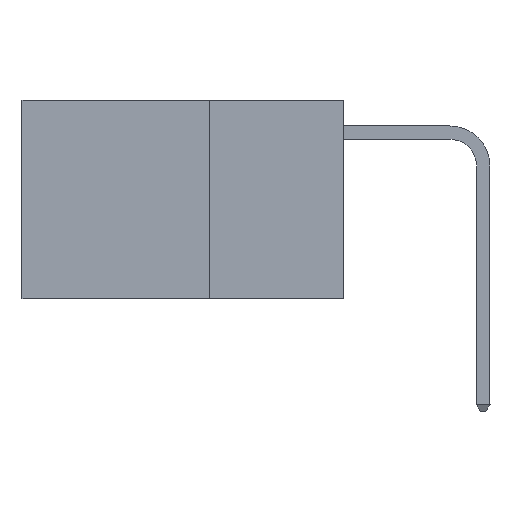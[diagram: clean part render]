
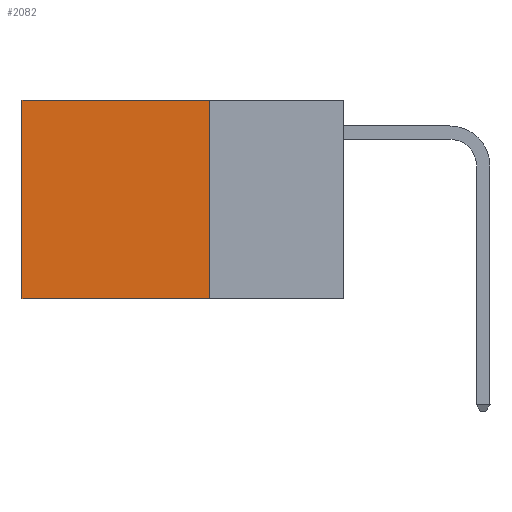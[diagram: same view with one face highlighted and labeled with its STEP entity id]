
A CAD part, left-side view. The second image highlights one B-rep face of the part: STEP entity #2082.
In plain terms, the highlighted planar face has unit normal (-1, 0, 0).
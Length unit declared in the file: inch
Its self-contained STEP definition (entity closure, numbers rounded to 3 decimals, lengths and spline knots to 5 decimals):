
#79 = EDGE_LOOP ( 'NONE', ( #1458, #371, #5404, #11312 ) ) ;
#185 = VECTOR ( 'NONE', #7376, 39.37008 ) ;
#190 = DIRECTION ( 'NONE',  ( 0., 1., 0. ) ) ;
#327 = LINE ( 'NONE', #8864, #5512 ) ;
#371 = ORIENTED_EDGE ( 'NONE', *, *, #4762, .F. ) ;
#1458 = ORIENTED_EDGE ( 'NONE', *, *, #11889, .T. ) ;
#1567 = CARTESIAN_POINT ( 'NONE',  ( 0.2625, 0.6, -0.37 ) ) ;
#1612 = EDGE_CURVE ( 'NONE', #6761, #1653, #1782, .T. ) ;
#1653 = VERTEX_POINT ( 'NONE', #11416 ) ;
#1782 = LINE ( 'NONE', #2996, #12418 ) ;
#1941 = PLANE ( 'NONE',  #12391 ) ;
#2082 = ADVANCED_FACE ( 'NONE', ( #6788 ), #1941, .F. ) ;
#2513 = VECTOR ( 'NONE', #2776, 39.37008 ) ;
#2776 = DIRECTION ( 'NONE',  ( 0., 0., -1. ) ) ;
#2996 = CARTESIAN_POINT ( 'NONE',  ( 0.2625, 0.25, 0. ) ) ;
#3044 = CARTESIAN_POINT ( 'NONE',  ( 0.2625, 0.25, -0.37 ) ) ;
#3886 = LINE ( 'NONE', #6598, #2513 ) ;
#4762 = EDGE_CURVE ( 'NONE', #7050, #7420, #327, .T. ) ;
#5024 = DIRECTION ( 'NONE',  ( 1., 0., 0. ) ) ;
#5359 = EDGE_CURVE ( 'NONE', #6761, #7050, #3886, .T. ) ;
#5404 = ORIENTED_EDGE ( 'NONE', *, *, #5359, .F. ) ;
#5512 = VECTOR ( 'NONE', #190, 39.37008 ) ;
#5626 = DIRECTION ( 'NONE',  ( 0., 1., 0. ) ) ;
#6598 = CARTESIAN_POINT ( 'NONE',  ( 0.2625, 0.25, 0. ) ) ;
#6761 = VERTEX_POINT ( 'NONE', #11987 ) ;
#6788 = FACE_OUTER_BOUND ( 'NONE', #79, .T. ) ;
#7050 = VERTEX_POINT ( 'NONE', #3044 ) ;
#7376 = DIRECTION ( 'NONE',  ( 0., 0., -1. ) ) ;
#7420 = VERTEX_POINT ( 'NONE', #1567 ) ;
#8864 = CARTESIAN_POINT ( 'NONE',  ( 0.2625, 0.25, -0.37 ) ) ;
#9403 = LINE ( 'NONE', #12168, #185 ) ;
#10654 = CARTESIAN_POINT ( 'NONE',  ( 0.2625, 0.25, 0. ) ) ;
#10782 = DIRECTION ( 'NONE',  ( 0., 0., -1. ) ) ;
#11312 = ORIENTED_EDGE ( 'NONE', *, *, #1612, .T. ) ;
#11416 = CARTESIAN_POINT ( 'NONE',  ( 0.2625, 0.6, 0. ) ) ;
#11889 = EDGE_CURVE ( 'NONE', #1653, #7420, #9403, .T. ) ;
#11987 = CARTESIAN_POINT ( 'NONE',  ( 0.2625, 0.25, 0. ) ) ;
#12168 = CARTESIAN_POINT ( 'NONE',  ( 0.2625, 0.6, 0. ) ) ;
#12391 = AXIS2_PLACEMENT_3D ( 'NONE', #10654, #5024, #10782 ) ;
#12418 = VECTOR ( 'NONE', #5626, 39.37008 ) ;
